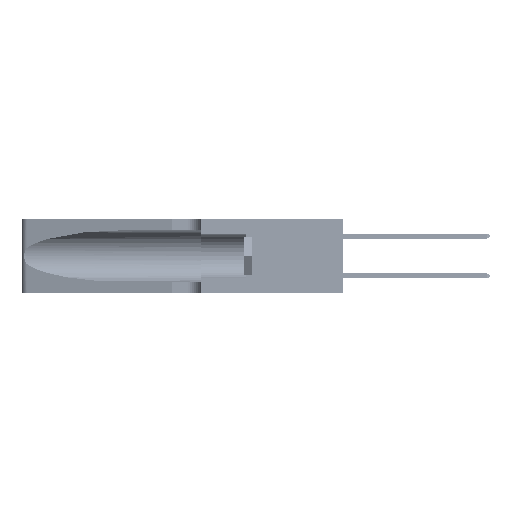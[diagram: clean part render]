
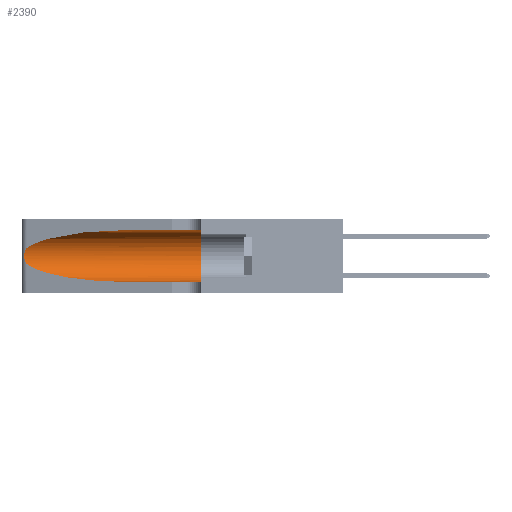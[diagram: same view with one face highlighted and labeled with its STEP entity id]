
A CAD part, left-side view. The second image highlights one B-rep face of the part: STEP entity #2390.
In plain terms, the highlighted cylindrical face has radius 3.308 mm (diameter 6.617 mm), a partial arc.
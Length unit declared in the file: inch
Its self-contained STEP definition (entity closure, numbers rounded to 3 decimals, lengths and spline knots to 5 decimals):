
#892 = VERTEX_POINT ( 'NONE', #41246 ) ;
#1506 = CYLINDRICAL_SURFACE ( 'NONE', #35114, 0.13025 ) ;
#1641 = CARTESIAN_POINT ( 'NONE',  ( 0.25487, 1.22718, 0.22369 ) ) ;
#2317 = CARTESIAN_POINT ( 'NONE',  ( 0.25787, 1.23484, 0.2124 ) ) ;
#2390 = ADVANCED_FACE ( 'NONE', ( #28559 ), #1506, .F. ) ;
#4261 = EDGE_CURVE ( 'NONE', #31826, #51947, #46241, .T. ) ;
#4740 = CARTESIAN_POINT ( 'NONE',  ( 0.1305, 0.72297, 0.05475 ) ) ;
#5714 = EDGE_CURVE ( 'NONE', #34762, #31826, #13298, .T. ) ;
#6913 = CARTESIAN_POINT ( 'NONE',  ( 0.2373, 1.15595, 0.08982 ) ) ;
#6997 = LINE ( 'NONE', #42019, #39138 ) ;
#9455 = DIRECTION ( 'NONE',  ( 0., -1., 0. ) ) ;
#10407 = EDGE_LOOP ( 'NONE', ( #40096, #28542, #50014, #46005, #47358, #14373 ) ) ;
#11127 = CARTESIAN_POINT ( 'NONE',  ( 0.1305, 0.72297, 0.05475 ) ) ;
#12937 = AXIS2_PLACEMENT_3D ( 'NONE', #44201, #40659, #16173 ) ;
#13298 =( BOUNDED_CURVE ( )  B_SPLINE_CURVE ( 3, ( #22645, #50828, #24198, #41870 ),
 .UNSPECIFIED., .F., .F. ) 
 B_SPLINE_CURVE_WITH_KNOTS ( ( 4, 4 ),
 ( 1.5708, 2.84003 ),
 .UNSPECIFIED. ) 
 CURVE ( )  GEOMETRIC_REPRESENTATION_ITEM ( )  RATIONAL_B_SPLINE_CURVE ( ( 1., 0.87, 0.87, 1. ) ) 
 REPRESENTATION_ITEM ( '' )  );
#14373 = ORIENTED_EDGE ( 'NONE', *, *, #19427, .F. ) ;
#16173 = DIRECTION ( 'NONE',  ( 0., 0., 1. ) ) ;
#17856 = CARTESIAN_POINT ( 'NONE',  ( 0.26018, 1.23835, 0.19895 ) ) ;
#17931 = CARTESIAN_POINT ( 'NONE',  ( 0.1305, 0.72297, 0.31525 ) ) ;
#18131 =( BOUNDED_CURVE ( )  B_SPLINE_CURVE ( 3, ( #51278, #6913, #30845, #11127 ),
 .UNSPECIFIED., .F., .T. ) 
 B_SPLINE_CURVE_WITH_KNOTS ( ( 4, 4 ),
 ( 3.44316, 4.71239 ),
 .UNSPECIFIED. ) 
 CURVE ( )  GEOMETRIC_REPRESENTATION_ITEM ( )  RATIONAL_B_SPLINE_CURVE ( ( 1., 0.87, 0.87, 1. ) ) 
 REPRESENTATION_ITEM ( '' )  );
#19427 = EDGE_CURVE ( 'NONE', #34762, #892, #6997, .T. ) ;
#20824 = VECTOR ( 'NONE', #9455, 39.37008 ) ;
#22393 = CARTESIAN_POINT ( 'NONE',  ( 0.25854, 1.2359, 0.20912 ) ) ;
#22645 = CARTESIAN_POINT ( 'NONE',  ( 0.1305, 0.72297, 0.31525 ) ) ;
#22687 = CARTESIAN_POINT ( 'NONE',  ( 0.1305, 0.35, 0.05475 ) ) ;
#24198 = CARTESIAN_POINT ( 'NONE',  ( 0.2373, 1.15595, 0.28018 ) ) ;
#26260 = CARTESIAN_POINT ( 'NONE',  ( 0.26017, 1.23833, 0.17102 ) ) ;
#27593 = VERTEX_POINT ( 'NONE', #22687 ) ;
#28542 = ORIENTED_EDGE ( 'NONE', *, *, #4261, .T. ) ;
#28559 = FACE_OUTER_BOUND ( 'NONE', #10407, .T. ) ;
#29797 = CARTESIAN_POINT ( 'NONE',  ( 0.25487, 1.22718, 0.14631 ) ) ;
#29971 = CARTESIAN_POINT ( 'NONE',  ( 0.25555, 1.22993, 0.14849 ) ) ;
#30009 = CARTESIAN_POINT ( 'NONE',  ( 0.1305, 1.61858, 0.05475 ) ) ;
#30142 = CARTESIAN_POINT ( 'NONE',  ( 0.25555, 1.22994, 0.2215 ) ) ;
#30293 = CARTESIAN_POINT ( 'NONE',  ( 0.25487, 1.22718, 0.14631 ) ) ;
#30490 = CARTESIAN_POINT ( 'NONE',  ( 0.26075, 1.23896, 0.19203 ) ) ;
#30845 = CARTESIAN_POINT ( 'NONE',  ( 0.18966, 0.96281, 0.05475 ) ) ;
#31030 = DIRECTION ( 'NONE',  ( 0., -1., 0. ) ) ;
#31200 = DIRECTION ( 'NONE',  ( 0., 0., -1. ) ) ;
#31826 = VERTEX_POINT ( 'NONE', #36170 ) ;
#34762 = VERTEX_POINT ( 'NONE', #17931 ) ;
#35114 = AXIS2_PLACEMENT_3D ( 'NONE', #51115, #31030, #31200 ) ;
#36170 = CARTESIAN_POINT ( 'NONE',  ( 0.25487, 1.22718, 0.22369 ) ) ;
#36900 = EDGE_CURVE ( 'NONE', #51947, #39429, #18131, .T. ) ;
#37618 = DIRECTION ( 'NONE',  ( 0., -1., 0. ) ) ;
#39138 = VECTOR ( 'NONE', #37618, 39.37008 ) ;
#39429 = VERTEX_POINT ( 'NONE', #4740 ) ;
#40096 = ORIENTED_EDGE ( 'NONE', *, *, #5714, .T. ) ;
#40659 = DIRECTION ( 'NONE',  ( 0., 1., 0. ) ) ;
#41246 = CARTESIAN_POINT ( 'NONE',  ( 0.1305, 0.35, 0.31525 ) ) ;
#41647 = LINE ( 'NONE', #30009, #20824 ) ;
#41870 = CARTESIAN_POINT ( 'NONE',  ( 0.25487, 1.22718, 0.22369 ) ) ;
#42019 = CARTESIAN_POINT ( 'NONE',  ( 0.1305, 1.61858, 0.31525 ) ) ;
#43393 = CARTESIAN_POINT ( 'NONE',  ( 0.25856, 1.23593, 0.16098 ) ) ;
#44201 = CARTESIAN_POINT ( 'NONE',  ( 0.1305, 0.35, 0.185 ) ) ;
#45861 = CARTESIAN_POINT ( 'NONE',  ( 0.26075, 1.23896, 0.178 ) ) ;
#46005 = ORIENTED_EDGE ( 'NONE', *, *, #51210, .T. ) ;
#46219 = CARTESIAN_POINT ( 'NONE',  ( 0.25639, 1.23184, 0.21858 ) ) ;
#46241 = B_SPLINE_CURVE_WITH_KNOTS ( 'NONE', 3,
 ( #1641, #30142, #46219, #2317, #22393, #17856, #30490, #45861, #26260, #43393, #49889, #50408, #29971, #29797 ),
 .UNSPECIFIED., .F., .F.,
 ( 4, 2, 2, 2, 2, 2, 4 ),
 ( 0., 0.00027, 0.00053, 0.00107, 0.0016, 0.00187, 0.00214 ),
 .UNSPECIFIED. ) ;
#47292 = EDGE_CURVE ( 'NONE', #892, #27593, #51407, .T. ) ;
#47358 = ORIENTED_EDGE ( 'NONE', *, *, #47292, .F. ) ;
#49889 = CARTESIAN_POINT ( 'NONE',  ( 0.25789, 1.23486, 0.15765 ) ) ;
#50014 = ORIENTED_EDGE ( 'NONE', *, *, #36900, .T. ) ;
#50408 = CARTESIAN_POINT ( 'NONE',  ( 0.25639, 1.23186, 0.15144 ) ) ;
#50828 = CARTESIAN_POINT ( 'NONE',  ( 0.18966, 0.96281, 0.31525 ) ) ;
#51115 = CARTESIAN_POINT ( 'NONE',  ( 0.1305, 1.61858, 0.185 ) ) ;
#51210 = EDGE_CURVE ( 'NONE', #39429, #27593, #41647, .T. ) ;
#51278 = CARTESIAN_POINT ( 'NONE',  ( 0.25487, 1.22718, 0.14631 ) ) ;
#51407 = CIRCLE ( 'NONE', #12937, 0.13025 ) ;
#51947 = VERTEX_POINT ( 'NONE', #30293 ) ;
